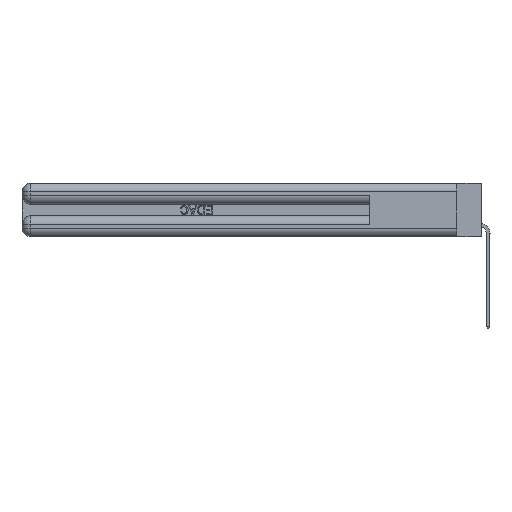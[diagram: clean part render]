
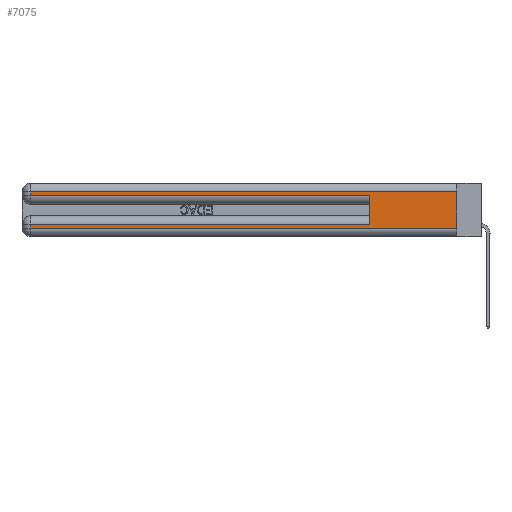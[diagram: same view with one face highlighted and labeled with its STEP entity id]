
A CAD part, left-side view. The second image highlights one B-rep face of the part: STEP entity #7075.
In plain terms, the highlighted planar face has unit normal (-1, 0, 0).
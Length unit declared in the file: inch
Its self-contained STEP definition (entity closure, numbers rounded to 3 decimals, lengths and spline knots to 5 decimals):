
#841 = VERTEX_POINT ( 'NONE', #35126 ) ;
#1190 = ORIENTED_EDGE ( 'NONE', *, *, #24050, .F. ) ;
#2051 = ORIENTED_EDGE ( 'NONE', *, *, #18243, .T. ) ;
#2358 = VECTOR ( 'NONE', #7279, 39.37008 ) ;
#3937 = LINE ( 'NONE', #26874, #30958 ) ;
#4707 = CARTESIAN_POINT ( 'NONE',  ( 0., 0., 0.06 ) ) ;
#5203 = CARTESIAN_POINT ( 'NONE',  ( 0., 0.6, 0.285 ) ) ;
#5462 = DIRECTION ( 'NONE',  ( 0., 1., 0. ) ) ;
#5463 = VERTEX_POINT ( 'NONE', #13988 ) ;
#5739 = VERTEX_POINT ( 'NONE', #5203 ) ;
#6084 = CARTESIAN_POINT ( 'NONE',  ( 0., 2.94, 0.37 ) ) ;
#7075 = ADVANCED_FACE ( 'NONE', ( #12277 ), #29312, .F. ) ;
#7279 = DIRECTION ( 'NONE',  ( 0., 0., 1. ) ) ;
#7581 = CARTESIAN_POINT ( 'NONE',  ( 0., 0., 0.37 ) ) ;
#10755 = EDGE_CURVE ( 'NONE', #26736, #841, #21804, .T. ) ;
#10915 = ORIENTED_EDGE ( 'NONE', *, *, #24201, .F. ) ;
#12277 = FACE_OUTER_BOUND ( 'NONE', #32687, .T. ) ;
#13883 = EDGE_CURVE ( 'NONE', #23709, #14502, #24134, .T. ) ;
#13988 = CARTESIAN_POINT ( 'NONE',  ( 0., 2.94, 0.285 ) ) ;
#14502 = VERTEX_POINT ( 'NONE', #4707 ) ;
#14633 = VECTOR ( 'NONE', #20641, 39.37008 ) ;
#15783 = VECTOR ( 'NONE', #30945, 39.37008 ) ;
#16257 = ORIENTED_EDGE ( 'NONE', *, *, #10755, .T. ) ;
#17710 = LINE ( 'NONE', #39594, #21023 ) ;
#18243 = EDGE_CURVE ( 'NONE', #5463, #5739, #17710, .T. ) ;
#19462 = DIRECTION ( 'NONE',  ( 0., -1., 0. ) ) ;
#19698 = VECTOR ( 'NONE', #19462, 39.37008 ) ;
#20641 = DIRECTION ( 'NONE',  ( 0., 0., -1. ) ) ;
#21023 = VECTOR ( 'NONE', #28532, 39.37008 ) ;
#21249 = CARTESIAN_POINT ( 'NONE',  ( 0., 0.6, 0.085 ) ) ;
#21659 = VECTOR ( 'NONE', #23289, 39.37008 ) ;
#21804 = LINE ( 'NONE', #30628, #15783 ) ;
#22197 = DIRECTION ( 'NONE',  ( 1., 0., 0. ) ) ;
#22796 = LINE ( 'NONE', #6084, #25032 ) ;
#23289 = DIRECTION ( 'NONE',  ( 0., 0., -1. ) ) ;
#23314 = LINE ( 'NONE', #27294, #2358 ) ;
#23450 = CARTESIAN_POINT ( 'NONE',  ( 0., 0., 0.37 ) ) ;
#23552 = EDGE_CURVE ( 'NONE', #26784, #23709, #22796, .T. ) ;
#23709 = VERTEX_POINT ( 'NONE', #39019 ) ;
#24050 = EDGE_CURVE ( 'NONE', #26736, #14502, #29372, .T. ) ;
#24124 = ORIENTED_EDGE ( 'NONE', *, *, #13883, .T. ) ;
#24134 = LINE ( 'NONE', #44430, #19698 ) ;
#24201 = EDGE_CURVE ( 'NONE', #27124, #5739, #23314, .T. ) ;
#24871 = ORIENTED_EDGE ( 'NONE', *, *, #28967, .T. ) ;
#25032 = VECTOR ( 'NONE', #27344, 39.37008 ) ;
#26736 = VERTEX_POINT ( 'NONE', #42386 ) ;
#26784 = VERTEX_POINT ( 'NONE', #42835 ) ;
#26874 = CARTESIAN_POINT ( 'NONE',  ( 0., 0., 0.085 ) ) ;
#27124 = VERTEX_POINT ( 'NONE', #21249 ) ;
#27294 = CARTESIAN_POINT ( 'NONE',  ( 0., 0.6, 0.145 ) ) ;
#27344 = DIRECTION ( 'NONE',  ( 0., 0., -1. ) ) ;
#28532 = DIRECTION ( 'NONE',  ( 0., -1., 0. ) ) ;
#28967 = EDGE_CURVE ( 'NONE', #841, #5463, #43809, .T. ) ;
#29312 = PLANE ( 'NONE',  #39086 ) ;
#29372 = LINE ( 'NONE', #23450, #21659 ) ;
#30589 = EDGE_CURVE ( 'NONE', #27124, #26784, #3937, .T. ) ;
#30628 = CARTESIAN_POINT ( 'NONE',  ( 0., 0., 0.31 ) ) ;
#30945 = DIRECTION ( 'NONE',  ( 0., 1., 0. ) ) ;
#30958 = VECTOR ( 'NONE', #5462, 39.37008 ) ;
#32224 = DIRECTION ( 'NONE',  ( 0., 0., -1. ) ) ;
#32531 = ORIENTED_EDGE ( 'NONE', *, *, #30589, .T. ) ;
#32687 = EDGE_LOOP ( 'NONE', ( #1190, #16257, #24871, #2051, #10915, #32531, #36544, #24124 ) ) ;
#35126 = CARTESIAN_POINT ( 'NONE',  ( 0., 2.94, 0.31 ) ) ;
#36544 = ORIENTED_EDGE ( 'NONE', *, *, #23552, .T. ) ;
#38660 = CARTESIAN_POINT ( 'NONE',  ( 0., 2.94, 0.37 ) ) ;
#39019 = CARTESIAN_POINT ( 'NONE',  ( 0., 2.94, 0.06 ) ) ;
#39086 = AXIS2_PLACEMENT_3D ( 'NONE', #7581, #22197, #32224 ) ;
#39594 = CARTESIAN_POINT ( 'NONE',  ( 0., 0., 0.285 ) ) ;
#42386 = CARTESIAN_POINT ( 'NONE',  ( 0., 0., 0.31 ) ) ;
#42835 = CARTESIAN_POINT ( 'NONE',  ( 0., 2.94, 0.085 ) ) ;
#43809 = LINE ( 'NONE', #38660, #14633 ) ;
#44430 = CARTESIAN_POINT ( 'NONE',  ( 0., 0., 0.06 ) ) ;
